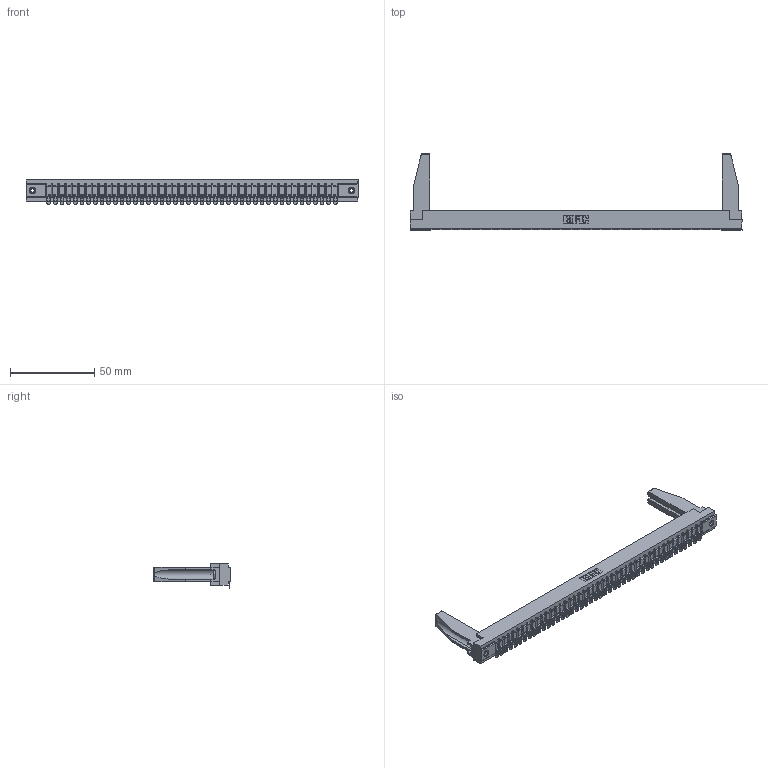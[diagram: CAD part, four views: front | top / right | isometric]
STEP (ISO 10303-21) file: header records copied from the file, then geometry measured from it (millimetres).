
FILE_DESCRIPTION (( 'STEP AP203' ), '1' );
FILE_NAME ('357-044-554-178.STEP', '2019-09-17T11:59:32', ( '' ), ( '' ), 'SwSTEP 2.0', 'SolidWorks 2016', '' );
FILE_SCHEMA (( 'CONFIG_CONTROL_DESIGN' ));
Length unit declared in the file: inch
Products named in the file (5): 307 Part_.156 Dia Mounting Holes; 307-290-002_554; 357-044-554-178; 307-220-078; 345-250-001_345-250-001-102
Assembly tree (49 placements, depth 2):
  357-044-554-178
    307 Part_.156 Dia Mounting Holes
    307-290-002_554  x44
    307-220-078  x2
    345-250-001_345-250-001-102  x2
Bounding box: 197.36 x 45.72 x 14.52 mm (x, y, z)
Volume: 25143.9 mm3; surface area: 30632.3 mm2
Topology: 49 solids, 49 shells, 3857 faces, 11785 edges, 7726 vertices
Faces by surface type: plane 2178, cylinder 1573, sphere 90, cone 12, torus 4
Entity records: 40878 total; most frequent: CARTESIAN_POINT 6896, ORIENTED_EDGE 6842, DIRECTION 6661, EDGE_CURVE 3421, VECTOR 2619, LINE 2619, VERTEX_POINT 2214, AXIS2_PLACEMENT_3D 2021
